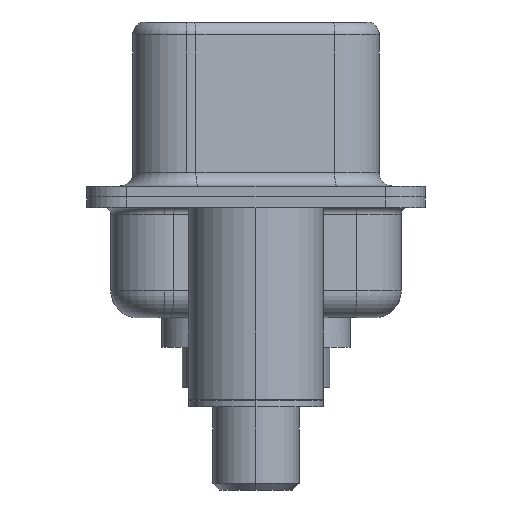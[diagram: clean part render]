
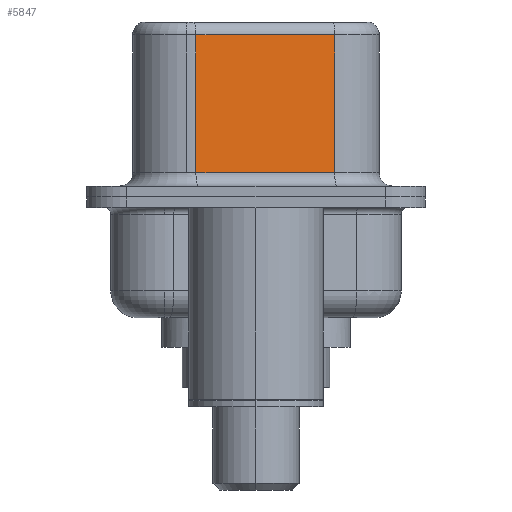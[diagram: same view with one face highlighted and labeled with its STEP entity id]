
A CAD part, left-side view. The second image highlights one B-rep face of the part: STEP entity #5847.
In plain terms, the highlighted planar face has unit normal (-0.985, -0.174, 0).
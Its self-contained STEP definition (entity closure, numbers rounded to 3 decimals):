
#231 = PLANE ( 'NONE',  #10633 ) ;
#519 = DIRECTION ( 'NONE',  ( -0.174, 0.985, 0. ) ) ;
#533 = DIRECTION ( 'NONE',  ( 0.985, 0.174, 0. ) ) ;
#975 = DIRECTION ( 'NONE',  ( 0., 0., -1. ) ) ;
#1092 = CARTESIAN_POINT ( 'NONE',  ( 4.565, -2.927, 6.52 ) ) ;
#2517 = CARTESIAN_POINT ( 'NONE',  ( 4.565, -2.927, 6.02 ) ) ;
#2685 = ORIENTED_EDGE ( 'NONE', *, *, #9601, .T. ) ;
#2796 = EDGE_CURVE ( 'NONE', #9564, #12550, #9309, .T. ) ;
#2974 = ORIENTED_EDGE ( 'NONE', *, *, #2796, .T. ) ;
#3314 = CARTESIAN_POINT ( 'NONE',  ( 4.565, -2.927, 0.9 ) ) ;
#3647 = ORIENTED_EDGE ( 'NONE', *, *, #11686, .T. ) ;
#3846 = VECTOR ( 'NONE', #10203, 1000. ) ;
#4314 = VECTOR ( 'NONE', #975, 1000. ) ;
#5253 = LINE ( 'NONE', #7905, #13248 ) ;
#5350 = CARTESIAN_POINT ( 'NONE',  ( 3.655, 2.233, 6.02 ) ) ;
#5528 = CARTESIAN_POINT ( 'NONE',  ( 3.655, 2.233, 6.52 ) ) ;
#5847 = ADVANCED_FACE ( 'NONE', ( #7244 ), #231, .F. ) ;
#6504 = LINE ( 'NONE', #5528, #8942 ) ;
#7244 = FACE_OUTER_BOUND ( 'NONE', #11218, .T. ) ;
#7820 = EDGE_CURVE ( 'NONE', #11697, #12550, #11996, .T. ) ;
#7863 = CARTESIAN_POINT ( 'NONE',  ( 3.655, 2.233, 0.9 ) ) ;
#7865 = CARTESIAN_POINT ( 'NONE',  ( 4.565, -2.927, 0.9 ) ) ;
#7905 = CARTESIAN_POINT ( 'NONE',  ( 4.565, -2.927, 6.02 ) ) ;
#8622 = VERTEX_POINT ( 'NONE', #5350 ) ;
#8942 = VECTOR ( 'NONE', #11808, 1000. ) ;
#9098 = ORIENTED_EDGE ( 'NONE', *, *, #7820, .F. ) ;
#9309 = LINE ( 'NONE', #3314, #3846 ) ;
#9564 = VERTEX_POINT ( 'NONE', #7863 ) ;
#9601 = EDGE_CURVE ( 'NONE', #11697, #8622, #5253, .T. ) ;
#10203 = DIRECTION ( 'NONE',  ( 0.174, -0.985, 0. ) ) ;
#10363 = CARTESIAN_POINT ( 'NONE',  ( 4.565, -2.927, 6.52 ) ) ;
#10633 = AXIS2_PLACEMENT_3D ( 'NONE', #1092, #533, #519 ) ;
#11218 = EDGE_LOOP ( 'NONE', ( #9098, #2685, #3647, #2974 ) ) ;
#11686 = EDGE_CURVE ( 'NONE', #8622, #9564, #6504, .T. ) ;
#11697 = VERTEX_POINT ( 'NONE', #2517 ) ;
#11808 = DIRECTION ( 'NONE',  ( 0., 0., -1. ) ) ;
#11996 = LINE ( 'NONE', #10363, #4314 ) ;
#12166 = DIRECTION ( 'NONE',  ( -0.174, 0.985, 0. ) ) ;
#12550 = VERTEX_POINT ( 'NONE', #7865 ) ;
#13248 = VECTOR ( 'NONE', #12166, 1000. ) ;
